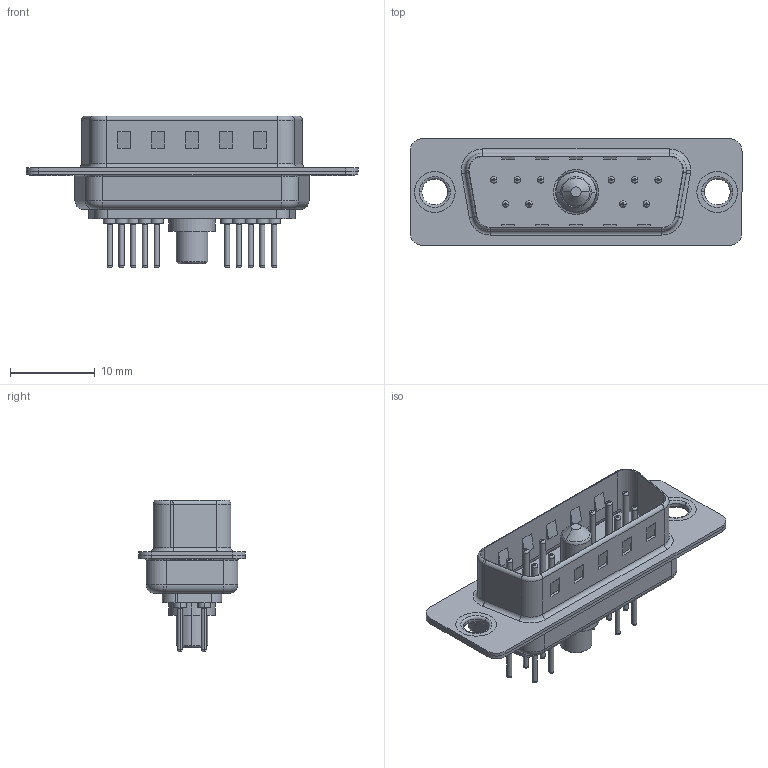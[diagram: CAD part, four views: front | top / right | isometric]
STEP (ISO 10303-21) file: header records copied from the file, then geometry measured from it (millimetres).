
FILE_DESCRIPTION (( 'STEP AP203' ), '1' );
FILE_NAME ('627-11W1224-4N1.STEP', '2019-05-25T12:34:27', ( '' ), ( '' ), 'SwSTEP 2.0', 'SolidWorks 2016', '' );
FILE_SCHEMA (( 'CONFIG_CONTROL_DESIGN' ));
Length unit declared in the file: millimetre
Products named in the file (8): Power Pin_40A S; 627Combo Contact Row 1_24; 627Combo Contact Row 2_24; 627-11W1224-4N1; 627Combo Housing_11W1; 627Combo Shell Rear_15 Contacts; 627Combo Shell Front_15 Contacts; 627Combo Thru Hole Rivet
Assembly tree (16 placements, depth 2):
  627-11W1224-4N1
    627Combo Housing_11W1
    627Combo Shell Rear_15 Contacts
    627Combo Shell Front_15 Contacts
    627Combo Thru Hole Rivet  x2
    Power Pin_40A S
    627Combo Contact Row 1_24  x6
    627Combo Contact Row 2_24  x4
Bounding box: 39.15 x 12.6 x 17.9 mm (x, y, z)
Volume: 1851.8 mm3; surface area: 4654.9 mm2
Topology: 17 solids, 20 shells, 737 faces, 1621 edges, 988 vertices
Faces by surface type: cylinder 280, plane 228, torus 220, cone 7, bspline 2
Entity records: 15205 total; most frequent: DIRECTION 2675, CARTESIAN_POINT 2452, ORIENTED_EDGE 2262, EDGE_CURVE 1131, AXIS2_PLACEMENT_3D 1061, VERTEX_POINT 708, EDGE_LOOP 581, CIRCLE 559
